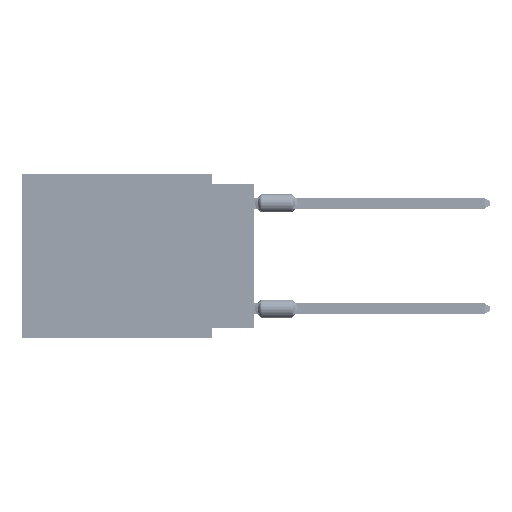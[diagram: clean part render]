
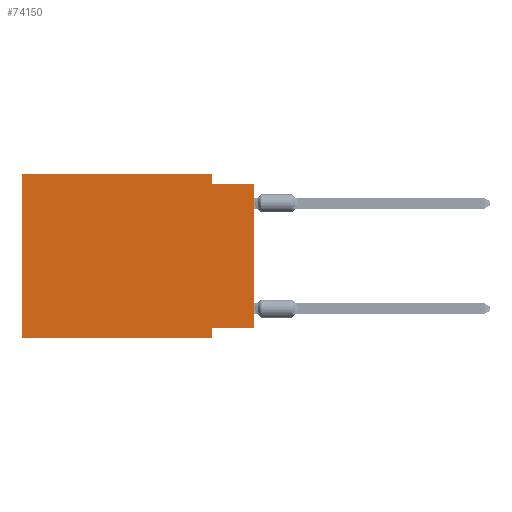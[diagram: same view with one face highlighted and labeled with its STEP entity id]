
A CAD part, left-side view. The second image highlights one B-rep face of the part: STEP entity #74150.
In plain terms, the highlighted planar face has unit normal (-1, 0, 0).
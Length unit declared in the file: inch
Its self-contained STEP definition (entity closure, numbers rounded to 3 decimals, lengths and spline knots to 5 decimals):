
#145 = DIRECTION ( 'NONE',  ( 1., 0., 0. ) ) ;
#1526 = VECTOR ( 'NONE', #75690, 39.37008 ) ;
#2684 = EDGE_CURVE ( 'NONE', #71031, #43402, #20039, .T. ) ;
#3677 = EDGE_CURVE ( 'NONE', #8383, #59712, #4910, .T. ) ;
#4699 = ORIENTED_EDGE ( 'NONE', *, *, #68952, .F. ) ;
#4910 = LINE ( 'NONE', #69551, #1526 ) ;
#5076 = LINE ( 'NONE', #17352, #29735 ) ;
#5808 = CARTESIAN_POINT ( 'NONE',  ( 0., 0., -0.025 ) ) ;
#6464 = CARTESIAN_POINT ( 'NONE',  ( 0., 0.1, -0.025 ) ) ;
#7290 = CARTESIAN_POINT ( 'NONE',  ( 0., 0.1, 0. ) ) ;
#7494 = DIRECTION ( 'NONE',  ( 0., -1., 0. ) ) ;
#8383 = VERTEX_POINT ( 'NONE', #6464 ) ;
#8905 = CARTESIAN_POINT ( 'NONE',  ( 0., 0.1, -0.39 ) ) ;
#9977 = CARTESIAN_POINT ( 'NONE',  ( 0., 0., -0.365 ) ) ;
#10919 = EDGE_CURVE ( 'NONE', #19039, #59712, #53535, .T. ) ;
#13554 = VECTOR ( 'NONE', #63165, 39.37008 ) ;
#17352 = CARTESIAN_POINT ( 'NONE',  ( 0., 0.1, 0. ) ) ;
#18207 = CARTESIAN_POINT ( 'NONE',  ( 0., 0.55, 0. ) ) ;
#19039 = VERTEX_POINT ( 'NONE', #9977 ) ;
#19767 = CARTESIAN_POINT ( 'NONE',  ( 0., 0.55, -0.39 ) ) ;
#20039 = LINE ( 'NONE', #8905, #46921 ) ;
#21840 = VERTEX_POINT ( 'NONE', #7290 ) ;
#25112 = CARTESIAN_POINT ( 'NONE',  ( 0., 0., -0.365 ) ) ;
#27388 = ORIENTED_EDGE ( 'NONE', *, *, #2684, .F. ) ;
#27970 = EDGE_LOOP ( 'NONE', ( #52671, #31122, #71153, #4699, #60052, #42696, #27388, #46635 ) ) ;
#28523 = DIRECTION ( 'NONE',  ( 0., 0., -1. ) ) ;
#29361 = DIRECTION ( 'NONE',  ( 0., 0., -1. ) ) ;
#29735 = VECTOR ( 'NONE', #28523, 39.37008 ) ;
#31122 = ORIENTED_EDGE ( 'NONE', *, *, #3677, .F. ) ;
#35976 = CARTESIAN_POINT ( 'NONE',  ( 0., 0.55, 0. ) ) ;
#42696 = ORIENTED_EDGE ( 'NONE', *, *, #68353, .T. ) ;
#43402 = VERTEX_POINT ( 'NONE', #65908 ) ;
#43970 = LINE ( 'NONE', #25112, #44226 ) ;
#44226 = VECTOR ( 'NONE', #54771, 39.37008 ) ;
#46635 = ORIENTED_EDGE ( 'NONE', *, *, #48441, .F. ) ;
#46921 = VECTOR ( 'NONE', #66639, 39.37008 ) ;
#48409 = VERTEX_POINT ( 'NONE', #54001 ) ;
#48441 = EDGE_CURVE ( 'NONE', #19039, #71031, #43970, .T. ) ;
#52671 = ORIENTED_EDGE ( 'NONE', *, *, #10919, .T. ) ;
#52919 = LINE ( 'NONE', #35976, #60829 ) ;
#53535 = LINE ( 'NONE', #71600, #58877 ) ;
#54001 = CARTESIAN_POINT ( 'NONE',  ( 0., 0.55, -0.39 ) ) ;
#54377 = PLANE ( 'NONE',  #63258 ) ;
#54771 = DIRECTION ( 'NONE',  ( 0., 1., 0. ) ) ;
#55289 = VECTOR ( 'NONE', #7494, 39.37008 ) ;
#56727 = CARTESIAN_POINT ( 'NONE',  ( 0., 0.55, 0. ) ) ;
#57671 = EDGE_CURVE ( 'NONE', #21840, #8383, #5076, .T. ) ;
#58877 = VECTOR ( 'NONE', #65843, 39.37008 ) ;
#59192 = VERTEX_POINT ( 'NONE', #56727 ) ;
#59457 = DIRECTION ( 'NONE',  ( 0., 0., 1. ) ) ;
#59536 = CARTESIAN_POINT ( 'NONE',  ( 0., 0.1, -0.365 ) ) ;
#59712 = VERTEX_POINT ( 'NONE', #5808 ) ;
#59780 = FACE_OUTER_BOUND ( 'NONE', #27970, .T. ) ;
#60052 = ORIENTED_EDGE ( 'NONE', *, *, #62967, .F. ) ;
#60829 = VECTOR ( 'NONE', #59457, 39.37008 ) ;
#62967 = EDGE_CURVE ( 'NONE', #48409, #59192, #52919, .T. ) ;
#63165 = DIRECTION ( 'NONE',  ( 0., -1., 0. ) ) ;
#63258 = AXIS2_PLACEMENT_3D ( 'NONE', #18207, #145, #29361 ) ;
#63909 = CARTESIAN_POINT ( 'NONE',  ( 0., 0.55, 0. ) ) ;
#65843 = DIRECTION ( 'NONE',  ( 0., 0., 1. ) ) ;
#65908 = CARTESIAN_POINT ( 'NONE',  ( 0., 0.1, -0.39 ) ) ;
#66639 = DIRECTION ( 'NONE',  ( 0., 0., -1. ) ) ;
#68353 = EDGE_CURVE ( 'NONE', #48409, #43402, #71749, .T. ) ;
#68552 = LINE ( 'NONE', #63909, #13554 ) ;
#68952 = EDGE_CURVE ( 'NONE', #59192, #21840, #68552, .T. ) ;
#69551 = CARTESIAN_POINT ( 'NONE',  ( 0., 0., -0.025 ) ) ;
#71031 = VERTEX_POINT ( 'NONE', #59536 ) ;
#71153 = ORIENTED_EDGE ( 'NONE', *, *, #57671, .F. ) ;
#71600 = CARTESIAN_POINT ( 'NONE',  ( 0., 0., 0. ) ) ;
#71749 = LINE ( 'NONE', #19767, #55289 ) ;
#74150 = ADVANCED_FACE ( 'NONE', ( #59780 ), #54377, .F. ) ;
#75690 = DIRECTION ( 'NONE',  ( 0., -1., 0. ) ) ;
